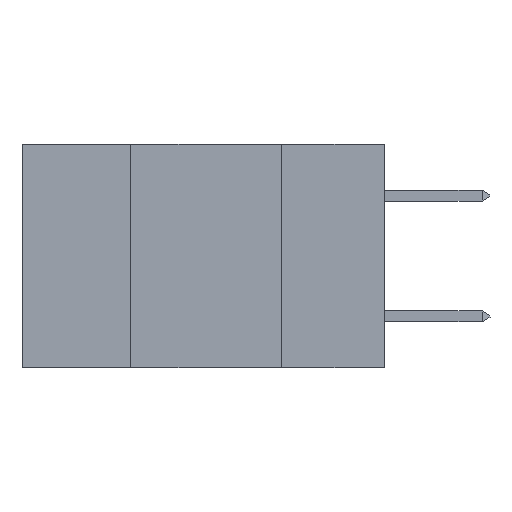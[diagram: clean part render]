
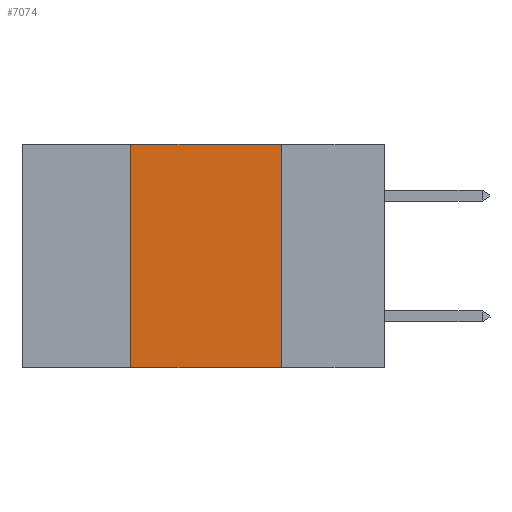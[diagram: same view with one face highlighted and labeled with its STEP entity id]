
A CAD part, left-side view. The second image highlights one B-rep face of the part: STEP entity #7074.
In plain terms, the highlighted planar face has unit normal (-1, 0, 0).
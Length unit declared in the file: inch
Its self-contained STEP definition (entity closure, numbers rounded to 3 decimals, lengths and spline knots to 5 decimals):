
#332 = DIRECTION ( 'NONE',  ( 0., 0., -1. ) ) ;
#333 = VECTOR ( 'NONE', #4212, 39.37008 ) ;
#614 = CARTESIAN_POINT ( 'NONE',  ( 0., 0.6, 0. ) ) ;
#1126 = CARTESIAN_POINT ( 'NONE',  ( 0., 0.6, -0.37 ) ) ;
#2901 = VERTEX_POINT ( 'NONE', #17090 ) ;
#3250 = EDGE_CURVE ( 'NONE', #19670, #2901, #14719, .T. ) ;
#4212 = DIRECTION ( 'NONE',  ( 0., -1., 0. ) ) ;
#4777 = LINE ( 'NONE', #11156, #21552 ) ;
#5499 = EDGE_LOOP ( 'NONE', ( #17398, #5595, #11643, #18216 ) ) ;
#5595 = ORIENTED_EDGE ( 'NONE', *, *, #3250, .F. ) ;
#5750 = PLANE ( 'NONE',  #12327 ) ;
#6579 = EDGE_CURVE ( 'NONE', #14721, #19670, #4777, .T. ) ;
#7074 = ADVANCED_FACE ( 'NONE', ( #7178 ), #5750, .F. ) ;
#7178 = FACE_OUTER_BOUND ( 'NONE', #5499, .T. ) ;
#8537 = EDGE_CURVE ( 'NONE', #2901, #9920, #21538, .T. ) ;
#9534 = DIRECTION ( 'NONE',  ( 0., 0., 1. ) ) ;
#9750 = CARTESIAN_POINT ( 'NONE',  ( 0., 0.42, 0. ) ) ;
#9920 = VERTEX_POINT ( 'NONE', #20869 ) ;
#10557 = LINE ( 'NONE', #1126, #17895 ) ;
#10838 = DIRECTION ( 'NONE',  ( 1., 0., 0. ) ) ;
#11076 = CARTESIAN_POINT ( 'NONE',  ( 0., 0.17, 0. ) ) ;
#11156 = CARTESIAN_POINT ( 'NONE',  ( 0., 0.42, 0. ) ) ;
#11643 = ORIENTED_EDGE ( 'NONE', *, *, #6579, .F. ) ;
#12327 = AXIS2_PLACEMENT_3D ( 'NONE', #17522, #10838, #332 ) ;
#14462 = DIRECTION ( 'NONE',  ( 0., 0., -1. ) ) ;
#14719 = LINE ( 'NONE', #614, #333 ) ;
#14721 = VERTEX_POINT ( 'NONE', #21895 ) ;
#15039 = DIRECTION ( 'NONE',  ( 0., -1., 0. ) ) ;
#17090 = CARTESIAN_POINT ( 'NONE',  ( 0., 0.17, 0. ) ) ;
#17224 = VECTOR ( 'NONE', #14462, 39.37008 ) ;
#17398 = ORIENTED_EDGE ( 'NONE', *, *, #8537, .F. ) ;
#17522 = CARTESIAN_POINT ( 'NONE',  ( 0., 0.6, 0. ) ) ;
#17895 = VECTOR ( 'NONE', #15039, 39.37008 ) ;
#18216 = ORIENTED_EDGE ( 'NONE', *, *, #21646, .T. ) ;
#19670 = VERTEX_POINT ( 'NONE', #9750 ) ;
#20869 = CARTESIAN_POINT ( 'NONE',  ( 0., 0.17, -0.37 ) ) ;
#21538 = LINE ( 'NONE', #11076, #17224 ) ;
#21552 = VECTOR ( 'NONE', #9534, 39.37008 ) ;
#21646 = EDGE_CURVE ( 'NONE', #14721, #9920, #10557, .T. ) ;
#21895 = CARTESIAN_POINT ( 'NONE',  ( 0., 0.42, -0.37 ) ) ;
